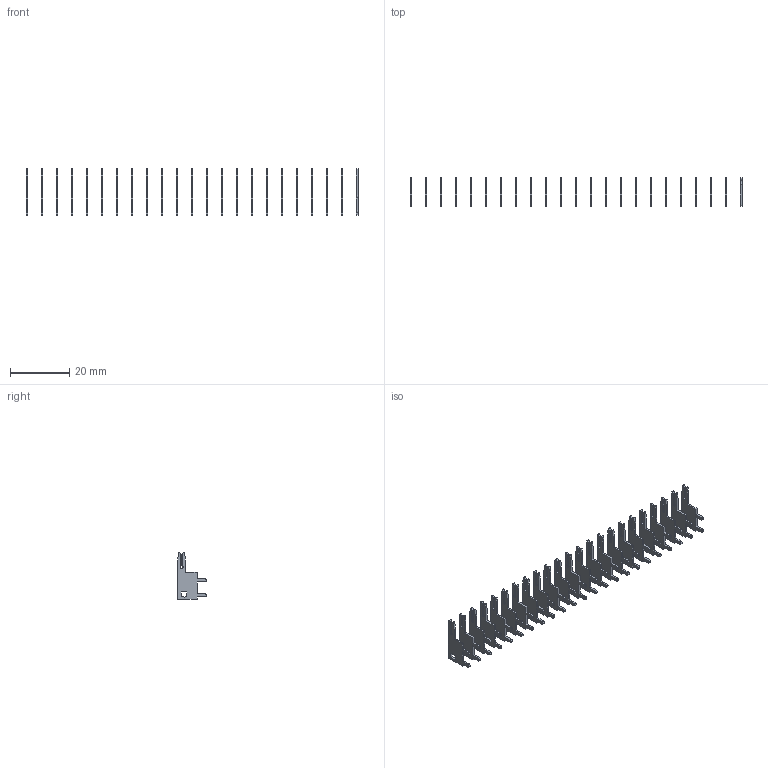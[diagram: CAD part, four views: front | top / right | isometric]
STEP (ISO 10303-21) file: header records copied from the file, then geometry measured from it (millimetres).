
FILE_DESCRIPTION (( 'STEP AP203' ), '1' );
FILE_NAME ('105-023-201-200.STEP', '2020-04-07T23:04:46', ( '' ), ( '' ), 'SwSTEP 2.0', 'SolidWorks 2016', '' );
FILE_SCHEMA (( 'CONFIG_CONTROL_DESIGN' ));
Length unit declared in the file: inch
Products named in the file (2): 100-290-001_100-290-201; 105-023-201-200
Assembly tree (23 placements, depth 2):
  105-023-201-200
    100-290-001_100-290-201  x23
Bounding box: 112.39 x 9.7 x 15.88 mm (x, y, z)
Volume: 1132.6 mm3; surface area: 4621.6 mm2
Topology: 23 solids, 23 shells, 805 faces, 2277 edges, 1518 vertices
Faces by surface type: plane 575, cylinder 230
Entity records: 2041 total; most frequent: CARTESIAN_POINT 238, DIRECTION 237, ORIENTED_EDGE 198, EDGE_CURVE 99, AXIS2_PLACEMENT_3D 81, VECTOR 75, LINE 75, VERTEX_POINT 66
